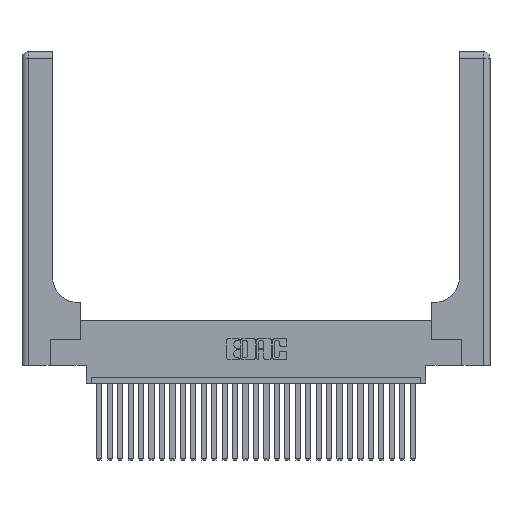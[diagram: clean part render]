
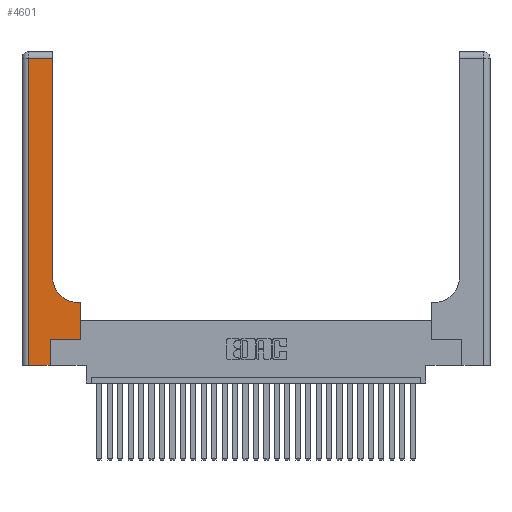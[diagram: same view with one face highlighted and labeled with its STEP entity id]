
A CAD part, top view. The second image highlights one B-rep face of the part: STEP entity #4601.
In plain terms, the highlighted planar face has unit normal (0, 0, 1).
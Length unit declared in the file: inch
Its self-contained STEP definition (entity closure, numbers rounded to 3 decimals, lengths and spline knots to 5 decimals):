
#143 = CARTESIAN_POINT ( 'NONE',  ( 0.2915, 2.94, 0.37 ) ) ;
#483 = VECTOR ( 'NONE', #10345, 39.37008 ) ;
#590 = VECTOR ( 'NONE', #1009, 39.37008 ) ;
#649 = VERTEX_POINT ( 'NONE', #15184 ) ;
#1009 = DIRECTION ( 'NONE',  ( 1., 0., 0. ) ) ;
#1241 = VECTOR ( 'NONE', #16888, 39.37008 ) ;
#1262 = EDGE_CURVE ( 'NONE', #14773, #15320, #17044, .T. ) ;
#1408 = CARTESIAN_POINT ( 'NONE',  ( 0.269, 0., 0.37 ) ) ;
#1559 = CARTESIAN_POINT ( 'NONE',  ( 0.5585, 0.25, 0.37 ) ) ;
#3199 = ORIENTED_EDGE ( 'NONE', *, *, #15402, .T. ) ;
#3208 = VECTOR ( 'NONE', #14991, 39.37008 ) ;
#3524 = FACE_OUTER_BOUND ( 'NONE', #11742, .T. ) ;
#3804 = EDGE_CURVE ( 'NONE', #13083, #26289, #27388, .T. ) ;
#3835 = LINE ( 'NONE', #24976, #8870 ) ;
#4601 = ADVANCED_FACE ( 'NONE', ( #3524 ), #16741, .F. ) ;
#4781 = CARTESIAN_POINT ( 'NONE',  ( 0.2915, 3., 0.37 ) ) ;
#5112 = CARTESIAN_POINT ( 'NONE',  ( 0.5585, 0.6, 0.37 ) ) ;
#5128 = EDGE_CURVE ( 'NONE', #6034, #24737, #20481, .T. ) ;
#5223 = DIRECTION ( 'NONE',  ( 0., 1., 0. ) ) ;
#5605 = EDGE_CURVE ( 'NONE', #24184, #13083, #3835, .T. ) ;
#5822 = CARTESIAN_POINT ( 'NONE',  ( 0.06, 3., 0.37 ) ) ;
#5853 = ORIENTED_EDGE ( 'NONE', *, *, #13738, .T. ) ;
#5936 = CARTESIAN_POINT ( 'NONE',  ( 0., 0., 0.37 ) ) ;
#6034 = VERTEX_POINT ( 'NONE', #1408 ) ;
#7035 = ORIENTED_EDGE ( 'NONE', *, *, #1262, .T. ) ;
#8870 = VECTOR ( 'NONE', #27290, 39.37008 ) ;
#9091 = VECTOR ( 'NONE', #22335, 39.37008 ) ;
#9734 = VERTEX_POINT ( 'NONE', #1559 ) ;
#10040 = ORIENTED_EDGE ( 'NONE', *, *, #5605, .T. ) ;
#10058 = CARTESIAN_POINT ( 'NONE',  ( 0., 3., 0.37 ) ) ;
#10345 = DIRECTION ( 'NONE',  ( 1., 0., 0. ) ) ;
#10696 = ORIENTED_EDGE ( 'NONE', *, *, #18796, .T. ) ;
#11420 = LINE ( 'NONE', #21718, #590 ) ;
#11742 = EDGE_LOOP ( 'NONE', ( #18160, #10040, #23117, #3199, #27007, #5853, #10696, #7035, #13689 ) ) ;
#13083 = VERTEX_POINT ( 'NONE', #28630 ) ;
#13338 = EDGE_CURVE ( 'NONE', #15320, #649, #16863, .T. ) ;
#13635 = CARTESIAN_POINT ( 'NONE',  ( 0.269, 0.25, 0.37 ) ) ;
#13689 = ORIENTED_EDGE ( 'NONE', *, *, #13338, .T. ) ;
#13738 = EDGE_CURVE ( 'NONE', #24737, #9734, #11420, .T. ) ;
#13855 = DIRECTION ( 'NONE',  ( 1., 0., 0. ) ) ;
#14478 = CARTESIAN_POINT ( 'NONE',  ( 0.5585, 0.25, 0.37 ) ) ;
#14773 = VERTEX_POINT ( 'NONE', #5112 ) ;
#14917 = LINE ( 'NONE', #5936, #483 ) ;
#14991 = DIRECTION ( 'NONE',  ( 0., -1., 0. ) ) ;
#15184 = CARTESIAN_POINT ( 'NONE',  ( 0.2915, 0.85, 0.37 ) ) ;
#15320 = VERTEX_POINT ( 'NONE', #21980 ) ;
#15402 = EDGE_CURVE ( 'NONE', #26289, #6034, #14917, .T. ) ;
#16328 = LINE ( 'NONE', #4781, #18860 ) ;
#16741 = PLANE ( 'NONE',  #17986 ) ;
#16863 = CIRCLE ( 'NONE', #18700, 0.25 ) ;
#16888 = DIRECTION ( 'NONE',  ( 0., 1., 0. ) ) ;
#17044 = LINE ( 'NONE', #24964, #9091 ) ;
#17166 = CARTESIAN_POINT ( 'NONE',  ( 0.06, 0., 0.37 ) ) ;
#17986 = AXIS2_PLACEMENT_3D ( 'NONE', #10058, #21399, #28675 ) ;
#18160 = ORIENTED_EDGE ( 'NONE', *, *, #23494, .T. ) ;
#18700 = AXIS2_PLACEMENT_3D ( 'NONE', #22850, #25169, #13855 ) ;
#18796 = EDGE_CURVE ( 'NONE', #9734, #14773, #25828, .T. ) ;
#18860 = VECTOR ( 'NONE', #20915, 39.37008 ) ;
#20481 = LINE ( 'NONE', #27927, #28416 ) ;
#20915 = DIRECTION ( 'NONE',  ( 0., 1., 0. ) ) ;
#21399 = DIRECTION ( 'NONE',  ( 0., 0., -1. ) ) ;
#21718 = CARTESIAN_POINT ( 'NONE',  ( 0.269, 0.25, 0.37 ) ) ;
#21980 = CARTESIAN_POINT ( 'NONE',  ( 0.5415, 0.6, 0.37 ) ) ;
#22335 = DIRECTION ( 'NONE',  ( -1., 0., 0. ) ) ;
#22850 = CARTESIAN_POINT ( 'NONE',  ( 0.5415, 0.85, 0.37 ) ) ;
#23117 = ORIENTED_EDGE ( 'NONE', *, *, #3804, .T. ) ;
#23494 = EDGE_CURVE ( 'NONE', #649, #24184, #16328, .T. ) ;
#24184 = VERTEX_POINT ( 'NONE', #143 ) ;
#24737 = VERTEX_POINT ( 'NONE', #13635 ) ;
#24964 = CARTESIAN_POINT ( 'NONE',  ( 0.2915, 0.6, 0.37 ) ) ;
#24976 = CARTESIAN_POINT ( 'NONE',  ( 0., 2.94, 0.37 ) ) ;
#25169 = DIRECTION ( 'NONE',  ( 0., 0., -1. ) ) ;
#25828 = LINE ( 'NONE', #14478, #1241 ) ;
#26289 = VERTEX_POINT ( 'NONE', #17166 ) ;
#27007 = ORIENTED_EDGE ( 'NONE', *, *, #5128, .T. ) ;
#27290 = DIRECTION ( 'NONE',  ( -1., 0., 0. ) ) ;
#27388 = LINE ( 'NONE', #5822, #3208 ) ;
#27927 = CARTESIAN_POINT ( 'NONE',  ( 0.269, 0., 0.37 ) ) ;
#28416 = VECTOR ( 'NONE', #5223, 39.37008 ) ;
#28630 = CARTESIAN_POINT ( 'NONE',  ( 0.06, 2.94, 0.37 ) ) ;
#28675 = DIRECTION ( 'NONE',  ( -1., 0., 0. ) ) ;
